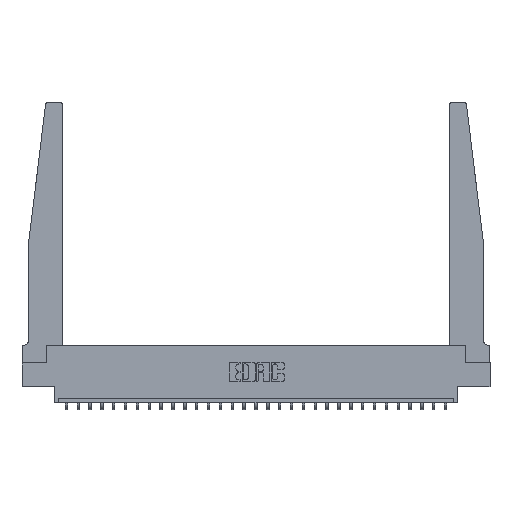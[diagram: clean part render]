
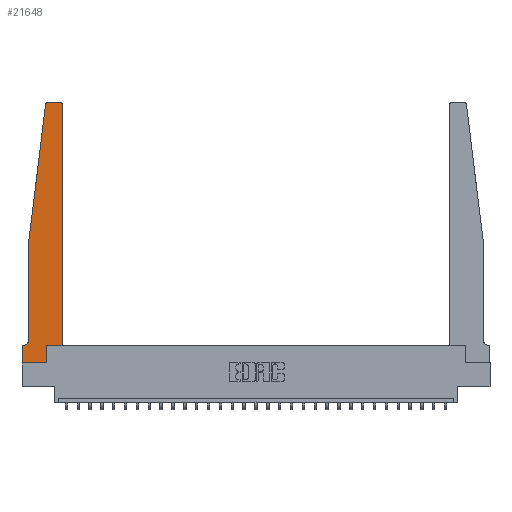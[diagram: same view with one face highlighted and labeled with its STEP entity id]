
A CAD part, top view. The second image highlights one B-rep face of the part: STEP entity #21648.
In plain terms, the highlighted planar face has unit normal (0, 0, 1).
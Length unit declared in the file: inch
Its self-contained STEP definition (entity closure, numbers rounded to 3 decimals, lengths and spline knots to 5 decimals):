
#192 = VERTEX_POINT ( 'NONE', #22466 ) ;
#273 = AXIS2_PLACEMENT_3D ( 'NONE', #13925, #24855, #3756 ) ;
#653 = CARTESIAN_POINT ( 'NONE',  ( 0.065, 1.25, 0.37 ) ) ;
#1271 = DIRECTION ( 'NONE',  ( 0., 1., 0. ) ) ;
#1579 = CIRCLE ( 'NONE', #273, 0.05 ) ;
#1651 = VECTOR ( 'NONE', #19903, 39.37008 ) ;
#1701 = EDGE_CURVE ( 'NONE', #2150, #22086, #22040, .T. ) ;
#2150 = VERTEX_POINT ( 'NONE', #2911 ) ;
#2568 = EDGE_LOOP ( 'NONE', ( #13391, #7012, #26484, #11225, #4871, #5179, #21986, #23325, #12114, #26091, #3013, #14280 ) ) ;
#2644 = CARTESIAN_POINT ( 'NONE',  ( 0.015, 0.1875, 0.37 ) ) ;
#2911 = CARTESIAN_POINT ( 'NONE',  ( 0.425, 0.18, 0.37 ) ) ;
#3013 = ORIENTED_EDGE ( 'NONE', *, *, #1701, .T. ) ;
#3110 = DIRECTION ( 'NONE',  ( 0., 0., 1. ) ) ;
#3310 = LINE ( 'NONE', #11463, #20510 ) ;
#3601 = CARTESIAN_POINT ( 'NONE',  ( 0., 0.1875, 0.37 ) ) ;
#3689 = VERTEX_POINT ( 'NONE', #14341 ) ;
#3756 = DIRECTION ( 'NONE',  ( -1., 0., 0. ) ) ;
#4268 = EDGE_CURVE ( 'NONE', #3689, #2150, #18850, .T. ) ;
#4683 = VERTEX_POINT ( 'NONE', #3601 ) ;
#4871 = ORIENTED_EDGE ( 'NONE', *, *, #24460, .T. ) ;
#5179 = ORIENTED_EDGE ( 'NONE', *, *, #24301, .T. ) ;
#5316 = VECTOR ( 'NONE', #1271, 39.37008 ) ;
#5335 = CARTESIAN_POINT ( 'NONE',  ( 0.395, 2.75, 0.37 ) ) ;
#5510 = VERTEX_POINT ( 'NONE', #19010 ) ;
#5703 = VECTOR ( 'NONE', #12081, 39.37008 ) ;
#5722 = EDGE_CURVE ( 'NONE', #5510, #11110, #3310, .T. ) ;
#5950 = CARTESIAN_POINT ( 'NONE',  ( 0.25, 2.75, 0.37 ) ) ;
#5972 = DIRECTION ( 'NONE',  ( 1., 0., 0. ) ) ;
#7005 = DIRECTION ( 'NONE',  ( 0., 0., 1. ) ) ;
#7012 = ORIENTED_EDGE ( 'NONE', *, *, #13242, .T. ) ;
#9207 = CARTESIAN_POINT ( 'NONE',  ( 0., 0., 0.37 ) ) ;
#11110 = VERTEX_POINT ( 'NONE', #653 ) ;
#11225 = ORIENTED_EDGE ( 'NONE', *, *, #15430, .T. ) ;
#11352 = CARTESIAN_POINT ( 'NONE',  ( 0.27653, 2.75, 0.37 ) ) ;
#11463 = CARTESIAN_POINT ( 'NONE',  ( 0.065, 1.25, 0.37 ) ) ;
#11501 = DIRECTION ( 'NONE',  ( 0., -1., 0. ) ) ;
#11619 = CARTESIAN_POINT ( 'NONE',  ( 0.2605, 0.18, 0.37 ) ) ;
#12081 = DIRECTION ( 'NONE',  ( 1., 0., 0. ) ) ;
#12114 = ORIENTED_EDGE ( 'NONE', *, *, #17741, .T. ) ;
#12933 = FACE_OUTER_BOUND ( 'NONE', #2568, .T. ) ;
#13096 = VECTOR ( 'NONE', #5972, 39.37008 ) ;
#13242 = EDGE_CURVE ( 'NONE', #20383, #5510, #14788, .T. ) ;
#13334 = DIRECTION ( 'NONE',  ( 1., 0., 0. ) ) ;
#13391 = ORIENTED_EDGE ( 'NONE', *, *, #22243, .T. ) ;
#13578 = DIRECTION ( 'NONE',  ( 1., 0., 0. ) ) ;
#13802 = CARTESIAN_POINT ( 'NONE',  ( 0.065, 0.1875, 0.37 ) ) ;
#13925 = CARTESIAN_POINT ( 'NONE',  ( 0.015, 0.2375, 0.37 ) ) ;
#13994 = VECTOR ( 'NONE', #11501, 39.37008 ) ;
#14053 = DIRECTION ( 'NONE',  ( -0.122, -0.992, 0. ) ) ;
#14126 = LINE ( 'NONE', #18348, #5703 ) ;
#14280 = ORIENTED_EDGE ( 'NONE', *, *, #26581, .T. ) ;
#14341 = CARTESIAN_POINT ( 'NONE',  ( 0.2605, 0.18, 0.37 ) ) ;
#14488 = CARTESIAN_POINT ( 'NONE',  ( 0.425, 0.18, 0.37 ) ) ;
#14788 = CIRCLE ( 'NONE', #23964, 0.03 ) ;
#14911 = AXIS2_PLACEMENT_3D ( 'NONE', #15515, #3110, #13578 ) ;
#15034 = DIRECTION ( 'NONE',  ( 1., 0., 0. ) ) ;
#15355 = CARTESIAN_POINT ( 'NONE',  ( 0.425, 0.18, 0.37 ) ) ;
#15430 = EDGE_CURVE ( 'NONE', #11110, #23541, #25170, .T. ) ;
#15515 = CARTESIAN_POINT ( 'NONE',  ( 0.395, 2.72, 0.37 ) ) ;
#15827 = CARTESIAN_POINT ( 'NONE',  ( 0.065, 0.2375, 0.37 ) ) ;
#16253 = DIRECTION ( 'NONE',  ( -1., 0., 0. ) ) ;
#16451 = CARTESIAN_POINT ( 'NONE',  ( 0., 0., 0.37 ) ) ;
#17741 = EDGE_CURVE ( 'NONE', #192, #3689, #24050, .T. ) ;
#18348 = CARTESIAN_POINT ( 'NONE',  ( 0., 0., 0.37 ) ) ;
#18477 = VERTEX_POINT ( 'NONE', #5335 ) ;
#18628 = VERTEX_POINT ( 'NONE', #16451 ) ;
#18850 = LINE ( 'NONE', #14488, #13096 ) ;
#19005 = DIRECTION ( 'NONE',  ( 0., 0., 1. ) ) ;
#19010 = CARTESIAN_POINT ( 'NONE',  ( 0.24675, 2.72367, 0.37 ) ) ;
#19492 = LINE ( 'NONE', #9207, #1651 ) ;
#19534 = CARTESIAN_POINT ( 'NONE',  ( 0.27653, 2.72, 0.37 ) ) ;
#19903 = DIRECTION ( 'NONE',  ( 0., -1., 0. ) ) ;
#20383 = VERTEX_POINT ( 'NONE', #11352 ) ;
#20510 = VECTOR ( 'NONE', #14053, 39.37008 ) ;
#20929 = VERTEX_POINT ( 'NONE', #2644 ) ;
#21648 = ADVANCED_FACE ( 'NONE', ( #12933 ), #21803, .T. ) ;
#21755 = VECTOR ( 'NONE', #26101, 39.37008 ) ;
#21803 = PLANE ( 'NONE',  #22482 ) ;
#21986 = ORIENTED_EDGE ( 'NONE', *, *, #25138, .T. ) ;
#22040 = LINE ( 'NONE', #15355, #25247 ) ;
#22086 = VERTEX_POINT ( 'NONE', #23901 ) ;
#22243 = EDGE_CURVE ( 'NONE', #18477, #20383, #24706, .T. ) ;
#22466 = CARTESIAN_POINT ( 'NONE',  ( 0.2605, 0., 0.37 ) ) ;
#22482 = AXIS2_PLACEMENT_3D ( 'NONE', #23577, #7005, #13334 ) ;
#23325 = ORIENTED_EDGE ( 'NONE', *, *, #26817, .T. ) ;
#23364 = VECTOR ( 'NONE', #16253, 39.37008 ) ;
#23541 = VERTEX_POINT ( 'NONE', #15827 ) ;
#23577 = CARTESIAN_POINT ( 'NONE',  ( 0., 0.1875, 0.37 ) ) ;
#23657 = LINE ( 'NONE', #13802, #21755 ) ;
#23901 = CARTESIAN_POINT ( 'NONE',  ( 0.425, 2.72, 0.37 ) ) ;
#23937 = DIRECTION ( 'NONE',  ( 0., 1., 0. ) ) ;
#23964 = AXIS2_PLACEMENT_3D ( 'NONE', #19534, #19005, #15034 ) ;
#24050 = LINE ( 'NONE', #11619, #5316 ) ;
#24301 = EDGE_CURVE ( 'NONE', #20929, #4683, #23657, .T. ) ;
#24460 = EDGE_CURVE ( 'NONE', #23541, #20929, #1579, .T. ) ;
#24495 = CIRCLE ( 'NONE', #14911, 0.03 ) ;
#24706 = LINE ( 'NONE', #5950, #23364 ) ;
#24855 = DIRECTION ( 'NONE',  ( 0., 0., -1. ) ) ;
#25138 = EDGE_CURVE ( 'NONE', #4683, #18628, #19492, .T. ) ;
#25170 = LINE ( 'NONE', #26114, #13994 ) ;
#25247 = VECTOR ( 'NONE', #23937, 39.37008 ) ;
#26091 = ORIENTED_EDGE ( 'NONE', *, *, #4268, .T. ) ;
#26101 = DIRECTION ( 'NONE',  ( -1., 0., 0. ) ) ;
#26114 = CARTESIAN_POINT ( 'NONE',  ( 0.065, 1.25, 0.37 ) ) ;
#26484 = ORIENTED_EDGE ( 'NONE', *, *, #5722, .T. ) ;
#26581 = EDGE_CURVE ( 'NONE', #22086, #18477, #24495, .T. ) ;
#26817 = EDGE_CURVE ( 'NONE', #18628, #192, #14126, .T. ) ;
